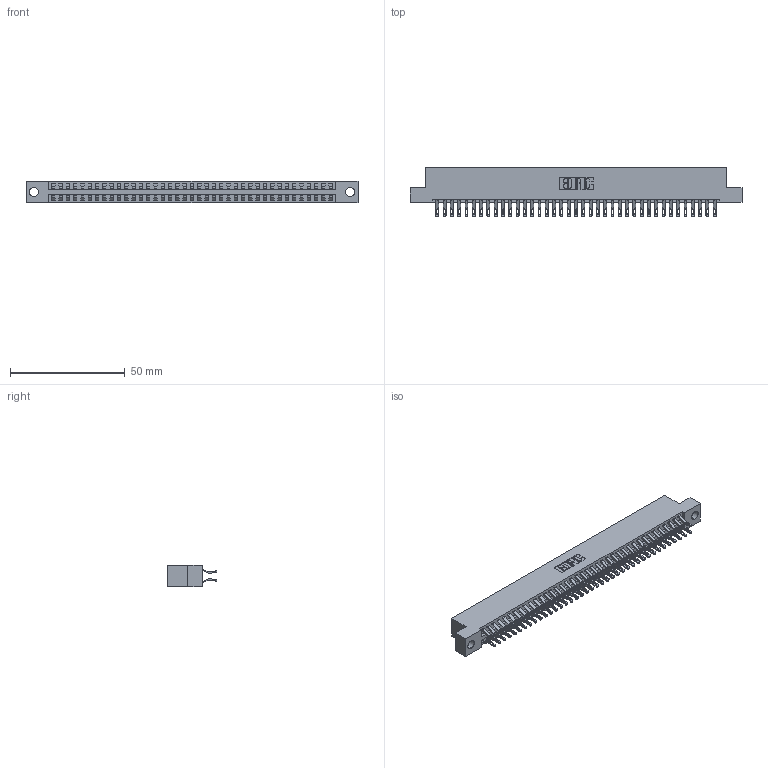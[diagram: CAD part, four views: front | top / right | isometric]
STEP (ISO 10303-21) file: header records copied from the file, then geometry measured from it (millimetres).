
FILE_DESCRIPTION (( 'STEP AP203' ), '1' );
FILE_NAME ('346-078-555-204.STEP', '2018-08-29T06:06:11', ( '' ), ( '' ), 'SwSTEP 2.0', 'SolidWorks 2016', '' );
FILE_SCHEMA (( 'CONFIG_CONTROL_DESIGN' ));
Length unit declared in the file: inch
Products named in the file (3): 345-292-001_555 Tail; 346-078-555-204; 346 Part_Flush Mounting Lugs - 0.156 Dia-TH
Assembly tree (79 placements, depth 2):
  346-078-555-204
    346 Part_Flush Mounting Lugs - 0.156 Dia-TH
    345-292-001_555 Tail  x78
Bounding box: 144.4 x 21.46 x 9.4 mm (x, y, z)
Volume: 14195.8 mm3; surface area: 20085.7 mm2
Topology: 79 solids, 79 shells, 4646 faces, 14603 edges, 9734 vertices
Faces by surface type: plane 2650, cylinder 1996
Entity records: 26185 total; most frequent: CARTESIAN_POINT 4354, ORIENTED_EDGE 4258, DIRECTION 3857, EDGE_CURVE 2129, LINE 1821, VECTOR 1821, VERTEX_POINT 1418, AXIS2_PLACEMENT_3D 1018
